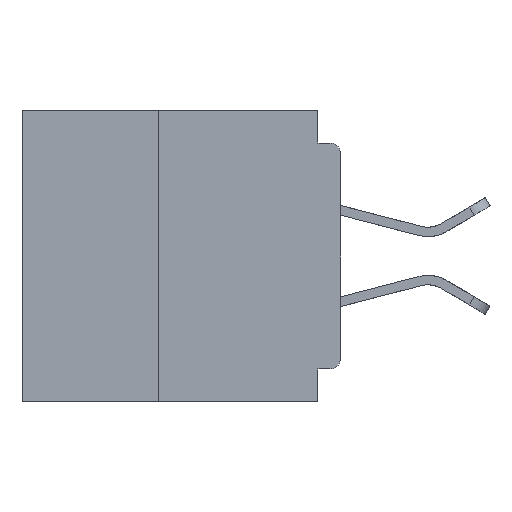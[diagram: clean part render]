
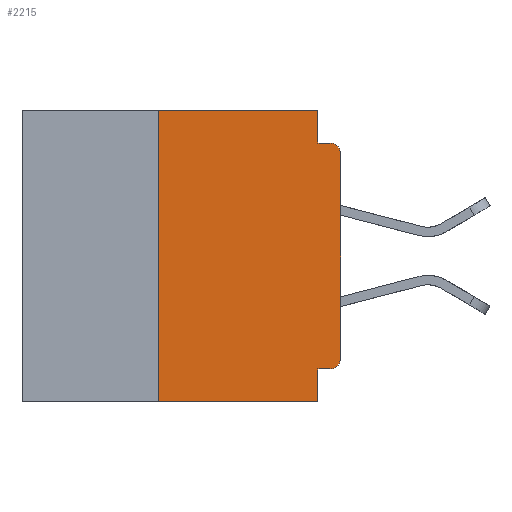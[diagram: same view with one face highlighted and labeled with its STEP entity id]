
A CAD part, left-side view. The second image highlights one B-rep face of the part: STEP entity #2215.
In plain terms, the highlighted planar face has unit normal (-1, 0, 0).
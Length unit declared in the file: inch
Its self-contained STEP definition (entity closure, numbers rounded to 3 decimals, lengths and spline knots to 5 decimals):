
#48 = CARTESIAN_POINT ( 'NONE',  ( 0., 0.437, -0.4 ) ) ;
#737 = DIRECTION ( 'NONE',  ( 0., -1., 0. ) ) ;
#956 = VERTEX_POINT ( 'NONE', #28570 ) ;
#1107 = VERTEX_POINT ( 'NONE', #23842 ) ;
#1253 = VERTEX_POINT ( 'NONE', #19048 ) ;
#1396 = CARTESIAN_POINT ( 'NONE',  ( 0., 0.031, -0.4 ) ) ;
#2215 = ADVANCED_FACE ( 'NONE', ( #25970 ), #32219, .F. ) ;
#2559 = CARTESIAN_POINT ( 'NONE',  ( 0., 0.437, 0. ) ) ;
#2893 = EDGE_CURVE ( 'NONE', #1107, #6571, #11360, .T. ) ;
#3592 = DIRECTION ( 'NONE',  ( 0., 0., 1. ) ) ;
#3724 = CARTESIAN_POINT ( 'NONE',  ( 0., 0.031, -0.045 ) ) ;
#3801 = EDGE_CURVE ( 'NONE', #14304, #956, #35318, .T. ) ;
#4611 = DIRECTION ( 'NONE',  ( 0., 0., -1. ) ) ;
#4763 = CARTESIAN_POINT ( 'NONE',  ( 0., 0.015, -0.045 ) ) ;
#6175 = EDGE_CURVE ( 'NONE', #6571, #18986, #9294, .T. ) ;
#6571 = VERTEX_POINT ( 'NONE', #8857 ) ;
#7298 = CARTESIAN_POINT ( 'NONE',  ( 0., 0.031, -0.4 ) ) ;
#7423 = VERTEX_POINT ( 'NONE', #1396 ) ;
#8077 = ORIENTED_EDGE ( 'NONE', *, *, #18855, .T. ) ;
#8857 = CARTESIAN_POINT ( 'NONE',  ( 0., 0.031, 0. ) ) ;
#9294 = LINE ( 'NONE', #16526, #30849 ) ;
#10019 = VECTOR ( 'NONE', #14766, 39.37008 ) ;
#10342 = VERTEX_POINT ( 'NONE', #27432 ) ;
#10669 = CARTESIAN_POINT ( 'NONE',  ( 0., 0., -0.355 ) ) ;
#11074 = ORIENTED_EDGE ( 'NONE', *, *, #2893, .F. ) ;
#11105 = DIRECTION ( 'NONE',  ( -1., 0., 0. ) ) ;
#11229 = CARTESIAN_POINT ( 'NONE',  ( 0., 0.015, -0.34 ) ) ;
#11360 = LINE ( 'NONE', #2559, #18094 ) ;
#11706 = DIRECTION ( 'NONE',  ( 0., -1., 0. ) ) ;
#12324 = CARTESIAN_POINT ( 'NONE',  ( 0., 0.437, 0. ) ) ;
#13073 = DIRECTION ( 'NONE',  ( -1., 0., 0. ) ) ;
#13268 = DIRECTION ( 'NONE',  ( 0., -1., 0. ) ) ;
#14304 = VERTEX_POINT ( 'NONE', #20675 ) ;
#14766 = DIRECTION ( 'NONE',  ( 0., 0., 1. ) ) ;
#14841 = LINE ( 'NONE', #27245, #35252 ) ;
#15159 = VERTEX_POINT ( 'NONE', #4763 ) ;
#15838 = DIRECTION ( 'NONE',  ( 0., 0., -1. ) ) ;
#16526 = CARTESIAN_POINT ( 'NONE',  ( 0., 0.031, 0. ) ) ;
#16709 = EDGE_LOOP ( 'NONE', ( #8077, #31548, #25305, #17380, #11074, #26441, #22387, #27861, #30780, #33665 ) ) ;
#16756 = AXIS2_PLACEMENT_3D ( 'NONE', #11229, #11105, #15838 ) ;
#16768 = DIRECTION ( 'NONE',  ( 0., 0., -1. ) ) ;
#17009 = AXIS2_PLACEMENT_3D ( 'NONE', #12324, #26098, #32303 ) ;
#17380 = ORIENTED_EDGE ( 'NONE', *, *, #6175, .F. ) ;
#18094 = VECTOR ( 'NONE', #737, 39.37008 ) ;
#18855 = EDGE_CURVE ( 'NONE', #956, #1253, #32425, .T. ) ;
#18950 = EDGE_CURVE ( 'NONE', #10342, #1107, #28951, .T. ) ;
#18986 = VERTEX_POINT ( 'NONE', #3724 ) ;
#19048 = CARTESIAN_POINT ( 'NONE',  ( 0., 0., -0.06 ) ) ;
#19097 = LINE ( 'NONE', #48, #32088 ) ;
#19638 = CIRCLE ( 'NONE', #32566, 0.015 ) ;
#19742 = VECTOR ( 'NONE', #27548, 39.37008 ) ;
#20601 = LINE ( 'NONE', #10669, #19742 ) ;
#20675 = CARTESIAN_POINT ( 'NONE',  ( 0., 0.015, -0.355 ) ) ;
#20816 = CARTESIAN_POINT ( 'NONE',  ( 0., 0.25, -0.4 ) ) ;
#21360 = EDGE_CURVE ( 'NONE', #18986, #15159, #14841, .T. ) ;
#21590 = VECTOR ( 'NONE', #3592, 39.37008 ) ;
#22387 = ORIENTED_EDGE ( 'NONE', *, *, #23857, .T. ) ;
#22661 = CARTESIAN_POINT ( 'NONE',  ( 0., 0.031, -0.355 ) ) ;
#23734 = VECTOR ( 'NONE', #4611, 39.37008 ) ;
#23842 = CARTESIAN_POINT ( 'NONE',  ( 0., 0.25, 0. ) ) ;
#23857 = EDGE_CURVE ( 'NONE', #10342, #7423, #19097, .T. ) ;
#25305 = ORIENTED_EDGE ( 'NONE', *, *, #21360, .F. ) ;
#25970 = FACE_OUTER_BOUND ( 'NONE', #16709, .T. ) ;
#26098 = DIRECTION ( 'NONE',  ( 1., 0., 0. ) ) ;
#26441 = ORIENTED_EDGE ( 'NONE', *, *, #18950, .F. ) ;
#27245 = CARTESIAN_POINT ( 'NONE',  ( 0., 0., -0.045 ) ) ;
#27432 = CARTESIAN_POINT ( 'NONE',  ( 0., 0.25, -0.4 ) ) ;
#27548 = DIRECTION ( 'NONE',  ( 0., 1., 0. ) ) ;
#27861 = ORIENTED_EDGE ( 'NONE', *, *, #33793, .F. ) ;
#28570 = CARTESIAN_POINT ( 'NONE',  ( 0., 0., -0.34 ) ) ;
#28607 = EDGE_CURVE ( 'NONE', #1253, #15159, #19638, .T. ) ;
#28694 = CARTESIAN_POINT ( 'NONE',  ( 0., 0., 0. ) ) ;
#28951 = LINE ( 'NONE', #20816, #21590 ) ;
#29824 = CARTESIAN_POINT ( 'NONE',  ( 0., 0.015, -0.06 ) ) ;
#30180 = VERTEX_POINT ( 'NONE', #22661 ) ;
#30780 = ORIENTED_EDGE ( 'NONE', *, *, #35424, .F. ) ;
#30849 = VECTOR ( 'NONE', #16768, 39.37008 ) ;
#31108 = LINE ( 'NONE', #7298, #23734 ) ;
#31548 = ORIENTED_EDGE ( 'NONE', *, *, #28607, .T. ) ;
#32088 = VECTOR ( 'NONE', #11706, 39.37008 ) ;
#32219 = PLANE ( 'NONE',  #17009 ) ;
#32303 = DIRECTION ( 'NONE',  ( 0., 0., -1. ) ) ;
#32425 = LINE ( 'NONE', #28694, #10019 ) ;
#32566 = AXIS2_PLACEMENT_3D ( 'NONE', #29824, #13073, #32618 ) ;
#32618 = DIRECTION ( 'NONE',  ( 0., 0., -1. ) ) ;
#33665 = ORIENTED_EDGE ( 'NONE', *, *, #3801, .T. ) ;
#33793 = EDGE_CURVE ( 'NONE', #30180, #7423, #31108, .T. ) ;
#35252 = VECTOR ( 'NONE', #13268, 39.37008 ) ;
#35318 = CIRCLE ( 'NONE', #16756, 0.015 ) ;
#35424 = EDGE_CURVE ( 'NONE', #14304, #30180, #20601, .T. ) ;
